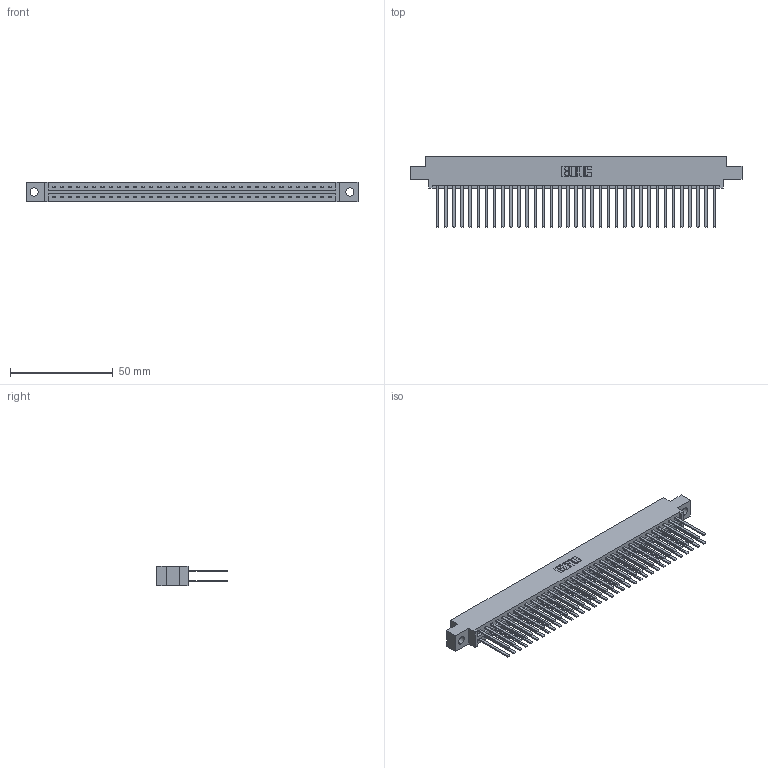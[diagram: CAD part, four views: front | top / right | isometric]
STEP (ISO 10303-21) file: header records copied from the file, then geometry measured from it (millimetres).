
FILE_DESCRIPTION (( 'STEP AP203' ), '1' );
FILE_NAME ('337-070-544-804.STEP', '2019-10-15T11:04:30', ( '' ), ( '' ), 'SwSTEP 2.0', 'SolidWorks 2016', '' );
FILE_SCHEMA (( 'CONFIG_CONTROL_DESIGN' ));
Length unit declared in the file: inch
Products named in the file (3): 337 Part_0.170 Offset - 0.156 Dia-TH; 345-292-001_345-293-144; 337-070-544-804
Assembly tree (71 placements, depth 2):
  337-070-544-804
    337 Part_0.170 Offset - 0.156 Dia-TH
    345-292-001_345-293-144  x70
Bounding box: 161.7 x 34.3 x 9.4 mm (x, y, z)
Volume: 17723.6 mm3; surface area: 23079.3 mm2
Topology: 71 solids, 71 shells, 3478 faces, 10333 edges, 6794 vertices
Faces by surface type: plane 2454, cylinder 1024
Entity records: 27993 total; most frequent: CARTESIAN_POINT 4722, ORIENTED_EDGE 4658, DIRECTION 4025, EDGE_CURVE 2329, LINE 2205, VECTOR 2205, VERTEX_POINT 1550, AXIS2_PLACEMENT_3D 910
